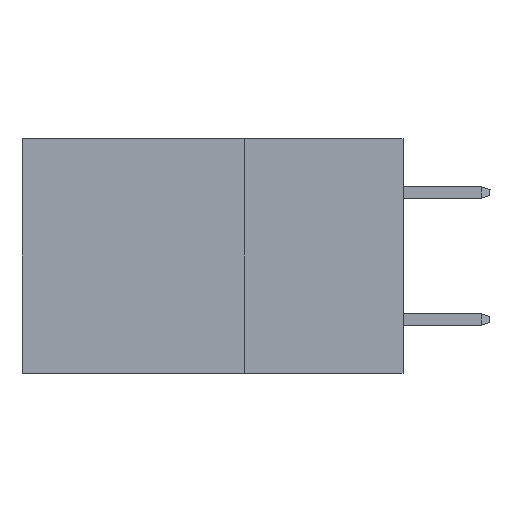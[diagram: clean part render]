
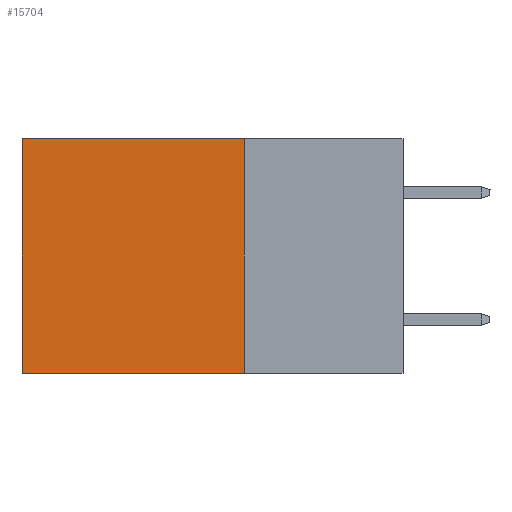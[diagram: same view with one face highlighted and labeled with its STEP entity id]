
A CAD part, left-side view. The second image highlights one B-rep face of the part: STEP entity #15704.
In plain terms, the highlighted planar face has unit normal (-1, 0, 0).
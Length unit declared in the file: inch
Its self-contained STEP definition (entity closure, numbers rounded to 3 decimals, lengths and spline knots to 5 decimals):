
#448 = CARTESIAN_POINT ( 'NONE',  ( 0.2875, 0.25, 0. ) ) ;
#2003 = ORIENTED_EDGE ( 'NONE', *, *, #24140, .F. ) ;
#2638 = DIRECTION ( 'NONE',  ( 0., 0., -1. ) ) ;
#2817 = VERTEX_POINT ( 'NONE', #25751 ) ;
#3757 = CARTESIAN_POINT ( 'NONE',  ( 0.2875, 0.25, 0. ) ) ;
#4013 = ORIENTED_EDGE ( 'NONE', *, *, #8526, .T. ) ;
#4726 = LINE ( 'NONE', #13902, #14069 ) ;
#5009 = VERTEX_POINT ( 'NONE', #7147 ) ;
#5193 = CARTESIAN_POINT ( 'NONE',  ( 0.2875, 0.25, 0. ) ) ;
#5295 = DIRECTION ( 'NONE',  ( 0., 1., 0. ) ) ;
#5477 = DIRECTION ( 'NONE',  ( 0., 0., -1. ) ) ;
#5512 = LINE ( 'NONE', #21295, #24478 ) ;
#6318 = EDGE_CURVE ( 'NONE', #2817, #9774, #5512, .T. ) ;
#6356 = EDGE_LOOP ( 'NONE', ( #19500, #2003, #7279, #4013 ) ) ;
#7147 = CARTESIAN_POINT ( 'NONE',  ( 0.2875, 0.25, -0.37 ) ) ;
#7279 = ORIENTED_EDGE ( 'NONE', *, *, #17675, .F. ) ;
#8526 = EDGE_CURVE ( 'NONE', #20308, #2817, #9814, .T. ) ;
#9413 = PLANE ( 'NONE',  #20018 ) ;
#9774 = VERTEX_POINT ( 'NONE', #26223 ) ;
#9814 = LINE ( 'NONE', #448, #23738 ) ;
#13902 = CARTESIAN_POINT ( 'NONE',  ( 0.2875, 0.25, -0.37 ) ) ;
#14069 = VECTOR ( 'NONE', #23075, 39.37008 ) ;
#15704 = ADVANCED_FACE ( 'NONE', ( #28245 ), #9413, .F. ) ;
#16486 = DIRECTION ( 'NONE',  ( 0., 0., -1. ) ) ;
#17180 = CARTESIAN_POINT ( 'NONE',  ( 0.2875, 0.25, 0. ) ) ;
#17234 = VECTOR ( 'NONE', #5477, 39.37008 ) ;
#17675 = EDGE_CURVE ( 'NONE', #20308, #5009, #24412, .T. ) ;
#19500 = ORIENTED_EDGE ( 'NONE', *, *, #6318, .T. ) ;
#20018 = AXIS2_PLACEMENT_3D ( 'NONE', #5193, #25979, #2638 ) ;
#20308 = VERTEX_POINT ( 'NONE', #3757 ) ;
#21295 = CARTESIAN_POINT ( 'NONE',  ( 0.2875, 0.6, 0. ) ) ;
#23075 = DIRECTION ( 'NONE',  ( 0., 1., 0. ) ) ;
#23738 = VECTOR ( 'NONE', #5295, 39.37008 ) ;
#24140 = EDGE_CURVE ( 'NONE', #5009, #9774, #4726, .T. ) ;
#24412 = LINE ( 'NONE', #17180, #17234 ) ;
#24478 = VECTOR ( 'NONE', #16486, 39.37008 ) ;
#25751 = CARTESIAN_POINT ( 'NONE',  ( 0.2875, 0.6, 0. ) ) ;
#25979 = DIRECTION ( 'NONE',  ( 1., 0., 0. ) ) ;
#26223 = CARTESIAN_POINT ( 'NONE',  ( 0.2875, 0.6, -0.37 ) ) ;
#28245 = FACE_OUTER_BOUND ( 'NONE', #6356, .T. ) ;
